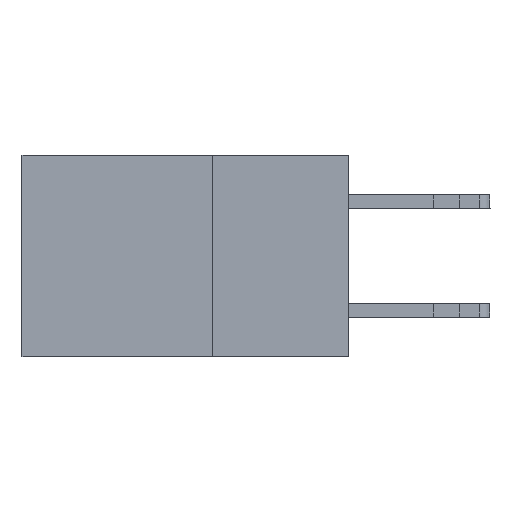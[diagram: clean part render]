
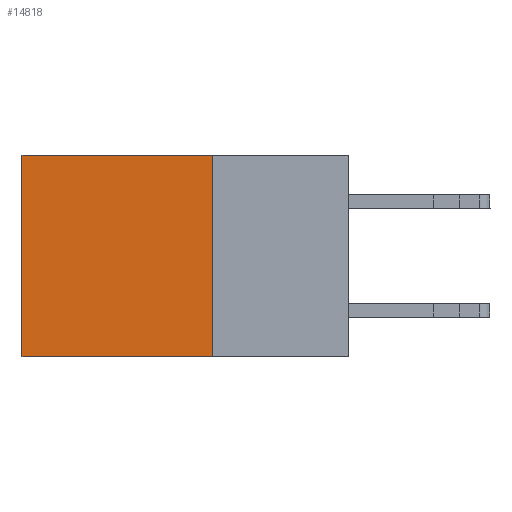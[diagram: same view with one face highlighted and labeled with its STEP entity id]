
A CAD part, left-side view. The second image highlights one B-rep face of the part: STEP entity #14818.
In plain terms, the highlighted planar face has unit normal (-1, 0, 0).
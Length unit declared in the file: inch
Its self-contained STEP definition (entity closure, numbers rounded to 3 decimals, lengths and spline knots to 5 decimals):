
#179 = LINE ( 'NONE', #11686, #13482 ) ;
#723 = PLANE ( 'NONE',  #8202 ) ;
#2260 = CARTESIAN_POINT ( 'NONE',  ( 0.2615, 0.6, 0. ) ) ;
#2361 = CARTESIAN_POINT ( 'NONE',  ( 0.2615, 0.6, -0.37 ) ) ;
#2501 = LINE ( 'NONE', #5124, #12777 ) ;
#2848 = ORIENTED_EDGE ( 'NONE', *, *, #12002, .F. ) ;
#3023 = ORIENTED_EDGE ( 'NONE', *, *, #8067, .T. ) ;
#3368 = VECTOR ( 'NONE', #12849, 39.37008 ) ;
#3842 = ORIENTED_EDGE ( 'NONE', *, *, #9236, .F. ) ;
#4460 = FACE_OUTER_BOUND ( 'NONE', #8147, .T. ) ;
#5073 = CARTESIAN_POINT ( 'NONE',  ( 0.2615, 0.6, -0.37 ) ) ;
#5124 = CARTESIAN_POINT ( 'NONE',  ( 0.2615, 0.25, -0.37 ) ) ;
#5909 = VERTEX_POINT ( 'NONE', #8199 ) ;
#6141 = CARTESIAN_POINT ( 'NONE',  ( 0.2615, 0.25, 0. ) ) ;
#6290 = DIRECTION ( 'NONE',  ( 0., 1., 0. ) ) ;
#6354 = LINE ( 'NONE', #2361, #3368 ) ;
#7093 = DIRECTION ( 'NONE',  ( 1., 0., 0. ) ) ;
#8067 = EDGE_CURVE ( 'NONE', #14004, #14871, #179, .T. ) ;
#8147 = EDGE_LOOP ( 'NONE', ( #10302, #3842, #2848, #3023 ) ) ;
#8199 = CARTESIAN_POINT ( 'NONE',  ( 0.2615, 0.25, -0.37 ) ) ;
#8202 = AXIS2_PLACEMENT_3D ( 'NONE', #11225, #7093, #16205 ) ;
#9236 = EDGE_CURVE ( 'NONE', #5909, #14483, #14886, .T. ) ;
#9928 = CARTESIAN_POINT ( 'NONE',  ( 0.2615, 0.25, -0.37 ) ) ;
#10047 = DIRECTION ( 'NONE',  ( 0., 0., -1. ) ) ;
#10302 = ORIENTED_EDGE ( 'NONE', *, *, #14418, .T. ) ;
#11225 = CARTESIAN_POINT ( 'NONE',  ( 0.2615, 0.25, -0.37 ) ) ;
#11686 = CARTESIAN_POINT ( 'NONE',  ( 0.2615, 0.25, 0. ) ) ;
#12002 = EDGE_CURVE ( 'NONE', #14004, #5909, #2501, .T. ) ;
#12432 = VECTOR ( 'NONE', #12535, 39.37008 ) ;
#12535 = DIRECTION ( 'NONE',  ( 0., 1., 0. ) ) ;
#12777 = VECTOR ( 'NONE', #10047, 39.37008 ) ;
#12849 = DIRECTION ( 'NONE',  ( 0., 0., -1. ) ) ;
#13482 = VECTOR ( 'NONE', #6290, 39.37008 ) ;
#14004 = VERTEX_POINT ( 'NONE', #6141 ) ;
#14418 = EDGE_CURVE ( 'NONE', #14871, #14483, #6354, .T. ) ;
#14483 = VERTEX_POINT ( 'NONE', #5073 ) ;
#14818 = ADVANCED_FACE ( 'NONE', ( #4460 ), #723, .F. ) ;
#14871 = VERTEX_POINT ( 'NONE', #2260 ) ;
#14886 = LINE ( 'NONE', #9928, #12432 ) ;
#16205 = DIRECTION ( 'NONE',  ( 0., 0., -1. ) ) ;
